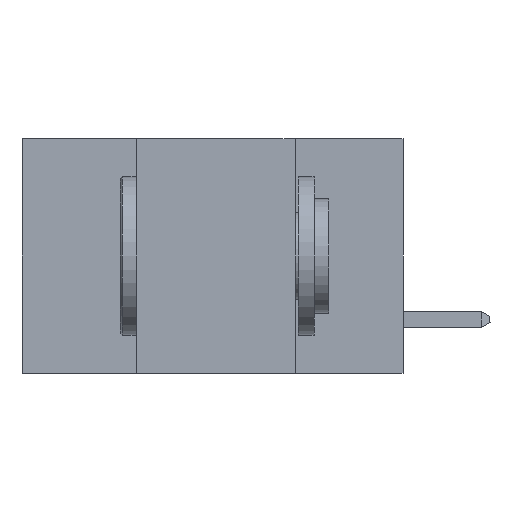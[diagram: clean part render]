
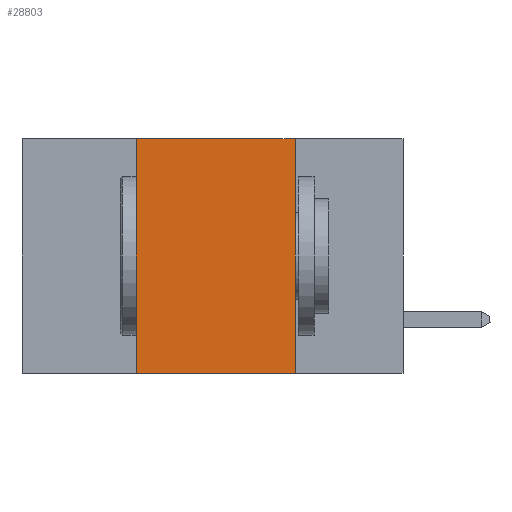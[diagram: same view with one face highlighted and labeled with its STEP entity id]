
A CAD part, left-side view. The second image highlights one B-rep face of the part: STEP entity #28803.
In plain terms, the highlighted planar face has unit normal (-1, 0, 0).
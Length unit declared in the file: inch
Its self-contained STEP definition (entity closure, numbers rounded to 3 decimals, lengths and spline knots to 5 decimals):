
#92 = ORIENTED_EDGE ( 'NONE', *, *, #16425, .T. ) ;
#227 = EDGE_CURVE ( 'NONE', #18543, #17877, #10241, .T. ) ;
#304 = LINE ( 'NONE', #23970, #10707 ) ;
#335 = VERTEX_POINT ( 'NONE', #19370 ) ;
#2258 = CARTESIAN_POINT ( 'NONE',  ( 0., 0.6, -0.37 ) ) ;
#4638 = LINE ( 'NONE', #20607, #24878 ) ;
#5139 = DIRECTION ( 'NONE',  ( 0., -1., 0. ) ) ;
#6986 = ORIENTED_EDGE ( 'NONE', *, *, #227, .F. ) ;
#8919 = CARTESIAN_POINT ( 'NONE',  ( 0., 0.17, 0. ) ) ;
#9085 = CARTESIAN_POINT ( 'NONE',  ( 0., 0.17, -0.37 ) ) ;
#9218 = FACE_OUTER_BOUND ( 'NONE', #15944, .T. ) ;
#10241 = LINE ( 'NONE', #16881, #11001 ) ;
#10432 = DIRECTION ( 'NONE',  ( 0., 0., 1. ) ) ;
#10707 = VECTOR ( 'NONE', #10432, 39.37008 ) ;
#10900 = EDGE_CURVE ( 'NONE', #335, #18543, #304, .T. ) ;
#11001 = VECTOR ( 'NONE', #28921, 39.37008 ) ;
#12438 = AXIS2_PLACEMENT_3D ( 'NONE', #21094, #25708, #30351 ) ;
#14011 = VECTOR ( 'NONE', #5139, 39.37008 ) ;
#15944 = EDGE_LOOP ( 'NONE', ( #19173, #6986, #22478, #92 ) ) ;
#16425 = EDGE_CURVE ( 'NONE', #335, #18393, #16556, .T. ) ;
#16556 = LINE ( 'NONE', #2258, #14011 ) ;
#16881 = CARTESIAN_POINT ( 'NONE',  ( 0., 0.6, 0. ) ) ;
#17154 = EDGE_CURVE ( 'NONE', #17877, #18393, #4638, .T. ) ;
#17877 = VERTEX_POINT ( 'NONE', #8919 ) ;
#18393 = VERTEX_POINT ( 'NONE', #9085 ) ;
#18543 = VERTEX_POINT ( 'NONE', #22421 ) ;
#18936 = DIRECTION ( 'NONE',  ( 0., 0., -1. ) ) ;
#19173 = ORIENTED_EDGE ( 'NONE', *, *, #17154, .F. ) ;
#19370 = CARTESIAN_POINT ( 'NONE',  ( 0., 0.42, -0.37 ) ) ;
#20607 = CARTESIAN_POINT ( 'NONE',  ( 0., 0.17, 0. ) ) ;
#20802 = PLANE ( 'NONE',  #12438 ) ;
#21094 = CARTESIAN_POINT ( 'NONE',  ( 0., 0.6, 0. ) ) ;
#22421 = CARTESIAN_POINT ( 'NONE',  ( 0., 0.42, 0. ) ) ;
#22478 = ORIENTED_EDGE ( 'NONE', *, *, #10900, .F. ) ;
#23970 = CARTESIAN_POINT ( 'NONE',  ( 0., 0.42, 0. ) ) ;
#24878 = VECTOR ( 'NONE', #18936, 39.37008 ) ;
#25708 = DIRECTION ( 'NONE',  ( 1., 0., 0. ) ) ;
#28803 = ADVANCED_FACE ( 'NONE', ( #9218 ), #20802, .F. ) ;
#28921 = DIRECTION ( 'NONE',  ( 0., -1., 0. ) ) ;
#30351 = DIRECTION ( 'NONE',  ( 0., 0., -1. ) ) ;
